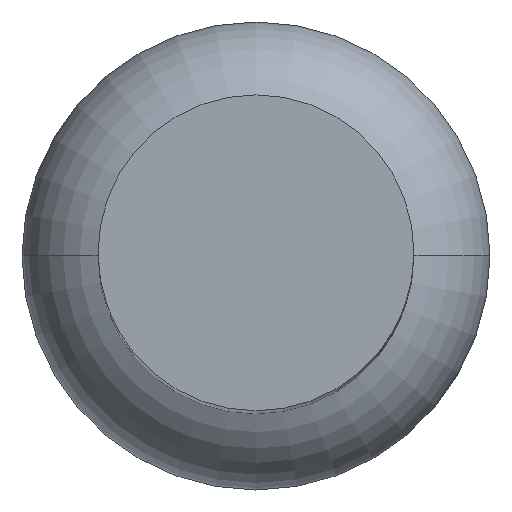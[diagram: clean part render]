
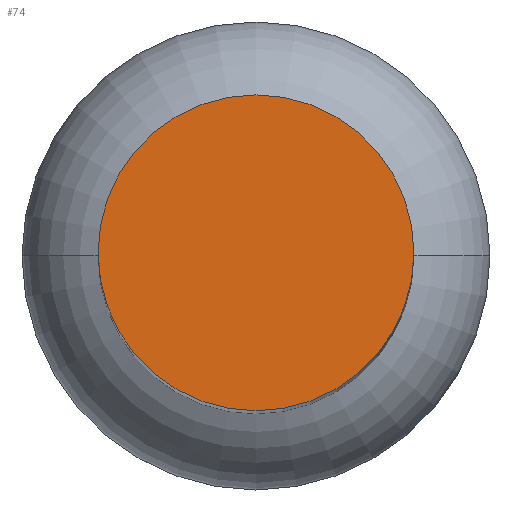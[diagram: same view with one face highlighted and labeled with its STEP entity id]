
A CAD part, top view. The second image highlights one B-rep face of the part: STEP entity #74.
In plain terms, the highlighted planar face has unit normal (0, 0, 1).
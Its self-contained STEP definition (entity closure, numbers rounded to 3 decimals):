
#35 = VERTEX_POINT ( 'NONE', #155 ) ;
#42 = DIRECTION ( 'NONE',  ( 1., 0., 0. ) ) ;
#46 = DIRECTION ( 'NONE',  ( 0., 0., -1. ) ) ;
#47 = CARTESIAN_POINT ( 'NONE',  ( 0., 0., 42.215 ) ) ;
#59 = AXIS2_PLACEMENT_3D ( 'NONE', #47, #46, #42 ) ;
#68 = PLANE ( 'NONE',  #107 ) ;
#72 = AXIS2_PLACEMENT_3D ( 'NONE', #254, #238, #241 ) ;
#74 = ADVANCED_FACE ( 'NONE', ( #144 ), #68, .F. ) ;
#100 = CARTESIAN_POINT ( 'NONE',  ( 0., 0., 42.215 ) ) ;
#107 = AXIS2_PLACEMENT_3D ( 'NONE', #100, #112, #109 ) ;
#108 = ORIENTED_EDGE ( 'NONE', *, *, #178, .F. ) ;
#109 = DIRECTION ( 'NONE',  ( 1., 0., 0. ) ) ;
#112 = DIRECTION ( 'NONE',  ( 0., 0., -1. ) ) ;
#126 = CARTESIAN_POINT ( 'NONE',  ( -3.429, 0., 42.215 ) ) ;
#141 = VERTEX_POINT ( 'NONE', #126 ) ;
#144 = FACE_OUTER_BOUND ( 'NONE', #224, .T. ) ;
#150 = EDGE_CURVE ( 'NONE', #35, #141, #165, .T. ) ;
#155 = CARTESIAN_POINT ( 'NONE',  ( 3.429, 0., 42.215 ) ) ;
#165 = CIRCLE ( 'NONE', #72, 3.429 ) ;
#178 = EDGE_CURVE ( 'NONE', #141, #35, #198, .T. ) ;
#198 = CIRCLE ( 'NONE', #59, 3.429 ) ;
#224 = EDGE_LOOP ( 'NONE', ( #108, #253 ) ) ;
#238 = DIRECTION ( 'NONE',  ( 0., 0., -1. ) ) ;
#241 = DIRECTION ( 'NONE',  ( 1., 0., 0. ) ) ;
#253 = ORIENTED_EDGE ( 'NONE', *, *, #150, .F. ) ;
#254 = CARTESIAN_POINT ( 'NONE',  ( 0., 0., 42.215 ) ) ;
